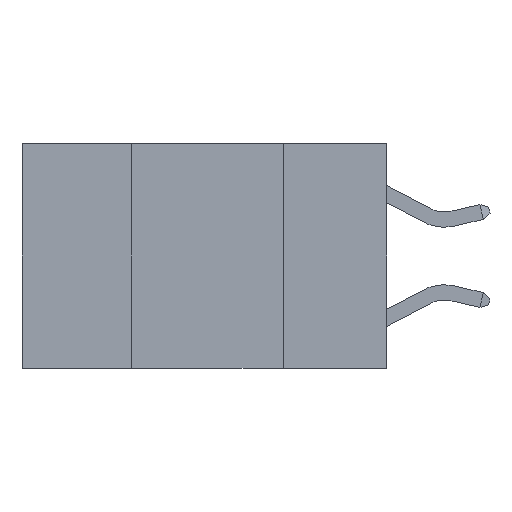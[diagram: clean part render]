
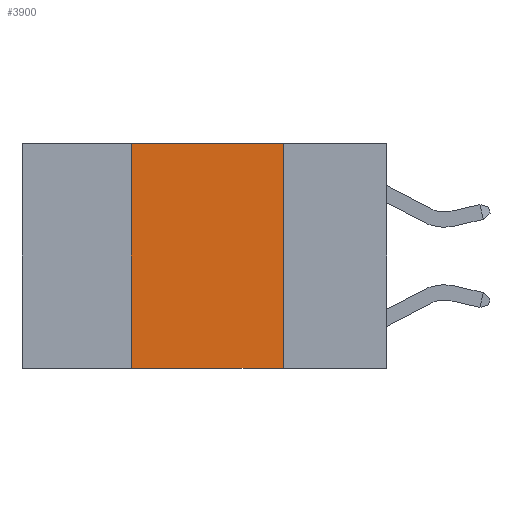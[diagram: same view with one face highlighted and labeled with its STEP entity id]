
A CAD part, left-side view. The second image highlights one B-rep face of the part: STEP entity #3900.
In plain terms, the highlighted planar face has unit normal (-1, 0, 0).
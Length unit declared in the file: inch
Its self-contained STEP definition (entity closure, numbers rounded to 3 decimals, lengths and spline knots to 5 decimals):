
#1493 = ORIENTED_EDGE ( 'NONE', *, *, #3265, .F. ) ;
#1607 = CARTESIAN_POINT ( 'NONE',  ( 0., 0.6, 0. ) ) ;
#1804 = VERTEX_POINT ( 'NONE', #3355 ) ;
#1952 = EDGE_CURVE ( 'NONE', #4361, #1804, #1980, .T. ) ;
#1980 = LINE ( 'NONE', #2743, #9158 ) ;
#2035 = EDGE_CURVE ( 'NONE', #4361, #7168, #8559, .T. ) ;
#2047 = EDGE_CURVE ( 'NONE', #7211, #1804, #2748, .T. ) ;
#2494 = VECTOR ( 'NONE', #6193, 39.37008 ) ;
#2743 = CARTESIAN_POINT ( 'NONE',  ( 0., 0.6, -0.37 ) ) ;
#2748 = LINE ( 'NONE', #4387, #8357 ) ;
#2830 = FACE_OUTER_BOUND ( 'NONE', #8222, .T. ) ;
#2969 = VECTOR ( 'NONE', #6014, 39.37008 ) ;
#3097 = DIRECTION ( 'NONE',  ( 1., 0., 0. ) ) ;
#3265 = EDGE_CURVE ( 'NONE', #7168, #7211, #4553, .T. ) ;
#3355 = CARTESIAN_POINT ( 'NONE',  ( 0., 0.17, -0.37 ) ) ;
#3900 = ADVANCED_FACE ( 'NONE', ( #2830 ), #6247, .F. ) ;
#3921 = ORIENTED_EDGE ( 'NONE', *, *, #2035, .F. ) ;
#4361 = VERTEX_POINT ( 'NONE', #7145 ) ;
#4372 = ORIENTED_EDGE ( 'NONE', *, *, #2047, .F. ) ;
#4387 = CARTESIAN_POINT ( 'NONE',  ( 0., 0.17, 0. ) ) ;
#4553 = LINE ( 'NONE', #1607, #2494 ) ;
#5220 = DIRECTION ( 'NONE',  ( 0., 0., -1. ) ) ;
#5500 = CARTESIAN_POINT ( 'NONE',  ( 0., 0.42, 0. ) ) ;
#6014 = DIRECTION ( 'NONE',  ( 0., 0., 1. ) ) ;
#6193 = DIRECTION ( 'NONE',  ( 0., -1., 0. ) ) ;
#6247 = PLANE ( 'NONE',  #7659 ) ;
#6955 = CARTESIAN_POINT ( 'NONE',  ( 0., 0.17, 0. ) ) ;
#7145 = CARTESIAN_POINT ( 'NONE',  ( 0., 0.42, -0.37 ) ) ;
#7156 = ORIENTED_EDGE ( 'NONE', *, *, #1952, .T. ) ;
#7168 = VERTEX_POINT ( 'NONE', #5500 ) ;
#7211 = VERTEX_POINT ( 'NONE', #6955 ) ;
#7576 = CARTESIAN_POINT ( 'NONE',  ( 0., 0.6, 0. ) ) ;
#7659 = AXIS2_PLACEMENT_3D ( 'NONE', #7576, #3097, #8238 ) ;
#7928 = DIRECTION ( 'NONE',  ( 0., -1., 0. ) ) ;
#8222 = EDGE_LOOP ( 'NONE', ( #4372, #1493, #3921, #7156 ) ) ;
#8238 = DIRECTION ( 'NONE',  ( 0., 0., -1. ) ) ;
#8357 = VECTOR ( 'NONE', #5220, 39.37008 ) ;
#8559 = LINE ( 'NONE', #9253, #2969 ) ;
#9158 = VECTOR ( 'NONE', #7928, 39.37008 ) ;
#9253 = CARTESIAN_POINT ( 'NONE',  ( 0., 0.42, 0. ) ) ;
